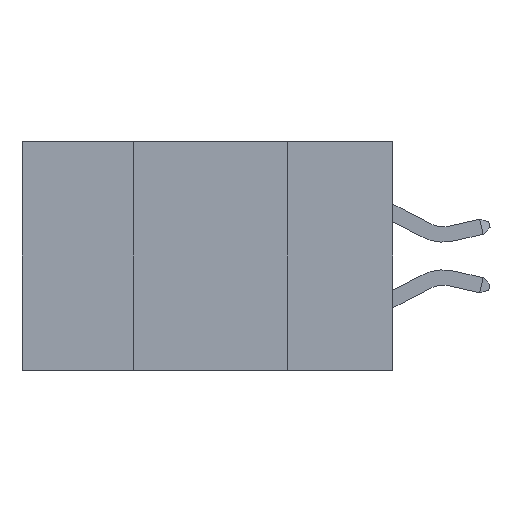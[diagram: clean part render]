
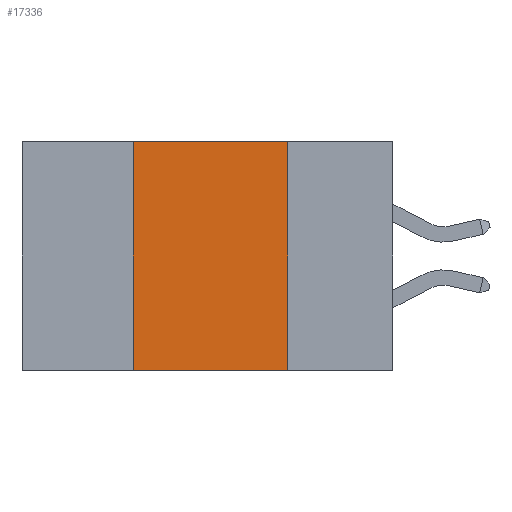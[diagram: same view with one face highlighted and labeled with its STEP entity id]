
A CAD part, left-side view. The second image highlights one B-rep face of the part: STEP entity #17336.
In plain terms, the highlighted planar face has unit normal (-1, 0, 0).
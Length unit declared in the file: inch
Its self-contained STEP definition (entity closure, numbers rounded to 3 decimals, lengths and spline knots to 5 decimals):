
#1149 = CARTESIAN_POINT ( 'NONE',  ( 0., 0.6, -0.37 ) ) ;
#1473 = ORIENTED_EDGE ( 'NONE', *, *, #25038, .T. ) ;
#1533 = CARTESIAN_POINT ( 'NONE',  ( 0., 0.6, 0. ) ) ;
#4149 = DIRECTION ( 'NONE',  ( 1., 0., 0. ) ) ;
#4886 = EDGE_LOOP ( 'NONE', ( #12178, #6478, #17034, #1473 ) ) ;
#6203 = EDGE_CURVE ( 'NONE', #16784, #25582, #22610, .T. ) ;
#6478 = ORIENTED_EDGE ( 'NONE', *, *, #15061, .F. ) ;
#6727 = AXIS2_PLACEMENT_3D ( 'NONE', #1533, #4149, #20811 ) ;
#8215 = VERTEX_POINT ( 'NONE', #10975 ) ;
#10348 = FACE_OUTER_BOUND ( 'NONE', #4886, .T. ) ;
#10738 = CARTESIAN_POINT ( 'NONE',  ( 0., 0.6, 0. ) ) ;
#10975 = CARTESIAN_POINT ( 'NONE',  ( 0., 0.17, -0.37 ) ) ;
#12157 = PLANE ( 'NONE',  #6727 ) ;
#12178 = ORIENTED_EDGE ( 'NONE', *, *, #25309, .F. ) ;
#13381 = CARTESIAN_POINT ( 'NONE',  ( 0., 0.17, 0. ) ) ;
#13580 = CARTESIAN_POINT ( 'NONE',  ( 0., 0.42, 0. ) ) ;
#14187 = VECTOR ( 'NONE', #16660, 39.37008 ) ;
#15061 = EDGE_CURVE ( 'NONE', #25582, #15520, #23286, .T. ) ;
#15520 = VERTEX_POINT ( 'NONE', #23653 ) ;
#16660 = DIRECTION ( 'NONE',  ( 0., 0., 1. ) ) ;
#16784 = VERTEX_POINT ( 'NONE', #21057 ) ;
#17034 = ORIENTED_EDGE ( 'NONE', *, *, #6203, .F. ) ;
#17336 = ADVANCED_FACE ( 'NONE', ( #10348 ), #12157, .F. ) ;
#18740 = CARTESIAN_POINT ( 'NONE',  ( 0., 0.42, 0. ) ) ;
#19142 = DIRECTION ( 'NONE',  ( 0., -1., 0. ) ) ;
#19846 = DIRECTION ( 'NONE',  ( 0., 0., -1. ) ) ;
#20811 = DIRECTION ( 'NONE',  ( 0., 0., -1. ) ) ;
#21057 = CARTESIAN_POINT ( 'NONE',  ( 0., 0.42, -0.37 ) ) ;
#22205 = LINE ( 'NONE', #13381, #24591 ) ;
#22610 = LINE ( 'NONE', #18740, #14187 ) ;
#23286 = LINE ( 'NONE', #10738, #23392 ) ;
#23392 = VECTOR ( 'NONE', #19142, 39.37008 ) ;
#23653 = CARTESIAN_POINT ( 'NONE',  ( 0., 0.17, 0. ) ) ;
#24148 = VECTOR ( 'NONE', #26390, 39.37008 ) ;
#24591 = VECTOR ( 'NONE', #19846, 39.37008 ) ;
#25038 = EDGE_CURVE ( 'NONE', #16784, #8215, #26673, .T. ) ;
#25309 = EDGE_CURVE ( 'NONE', #15520, #8215, #22205, .T. ) ;
#25582 = VERTEX_POINT ( 'NONE', #13580 ) ;
#26390 = DIRECTION ( 'NONE',  ( 0., -1., 0. ) ) ;
#26673 = LINE ( 'NONE', #1149, #24148 ) ;
